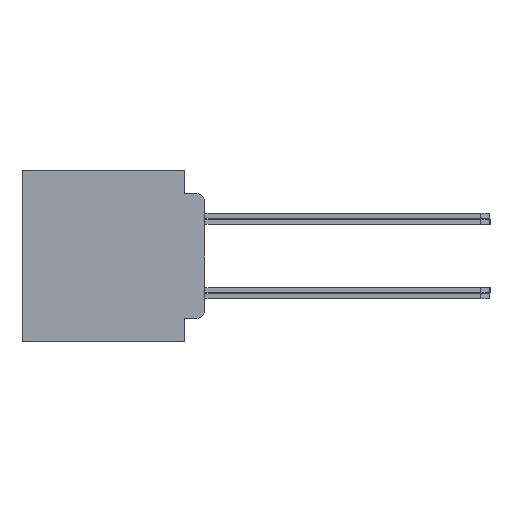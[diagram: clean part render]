
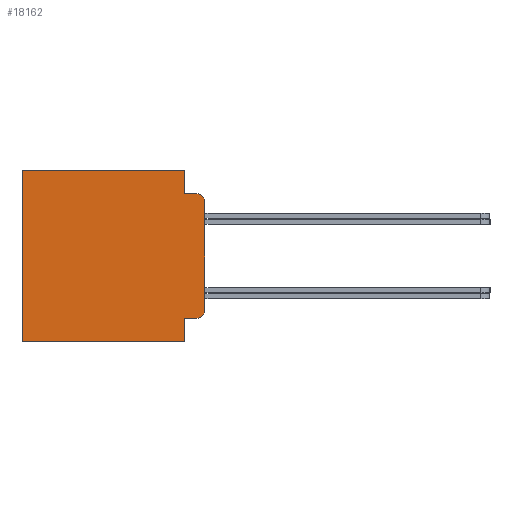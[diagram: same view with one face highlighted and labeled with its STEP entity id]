
A CAD part, left-side view. The second image highlights one B-rep face of the part: STEP entity #18162.
In plain terms, the highlighted planar face has unit normal (-1, 0, 0).
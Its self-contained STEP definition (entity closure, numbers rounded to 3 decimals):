
#563 = VERTEX_POINT ( 'NONE', #27452 ) ;
#600 = CARTESIAN_POINT ( 'NONE',  ( -67.462, 0., -5.486 ) ) ;
#1057 = EDGE_CURVE ( 'NONE', #22391, #24066, #13240, .T. ) ;
#1840 = LINE ( 'NONE', #24436, #25748 ) ;
#1884 = ORIENTED_EDGE ( 'NONE', *, *, #20820, .F. ) ;
#2280 = AXIS2_PLACEMENT_3D ( 'NONE', #17849, #24425, #22311 ) ;
#2644 = DIRECTION ( 'NONE',  ( 0., 1., 0. ) ) ;
#2706 = VERTEX_POINT ( 'NONE', #16538 ) ;
#3591 = LINE ( 'NONE', #10402, #8361 ) ;
#3735 = VECTOR ( 'NONE', #2644, 1000. ) ;
#3803 = AXIS2_PLACEMENT_3D ( 'NONE', #21195, #10219, #8195 ) ;
#3935 = CARTESIAN_POINT ( 'NONE',  ( -67.462, 1.295, 0. ) ) ;
#4358 = VERTEX_POINT ( 'NONE', #8052 ) ;
#4764 = ORIENTED_EDGE ( 'NONE', *, *, #26502, .T. ) ;
#4780 = ORIENTED_EDGE ( 'NONE', *, *, #1057, .F. ) ;
#5089 = CARTESIAN_POINT ( 'NONE',  ( -67.462, 0.508, -3.975 ) ) ;
#5610 = ORIENTED_EDGE ( 'NONE', *, *, #14342, .F. ) ;
#5852 = CIRCLE ( 'NONE', #2280, 0.508 ) ;
#6257 = ORIENTED_EDGE ( 'NONE', *, *, #21440, .F. ) ;
#6613 = CARTESIAN_POINT ( 'NONE',  ( -67.462, 11.684, -5.486 ) ) ;
#8052 = CARTESIAN_POINT ( 'NONE',  ( -67.462, 0., -3.467 ) ) ;
#8195 = DIRECTION ( 'NONE',  ( 0., 0., -1. ) ) ;
#8240 = VERTEX_POINT ( 'NONE', #24018 ) ;
#8361 = VECTOR ( 'NONE', #17074, 1000. ) ;
#8452 = VERTEX_POINT ( 'NONE', #5089 ) ;
#8797 = DIRECTION ( 'NONE',  ( 0., 0., -1. ) ) ;
#8942 = CARTESIAN_POINT ( 'NONE',  ( -67.462, 0., 5.486 ) ) ;
#9893 = CARTESIAN_POINT ( 'NONE',  ( -67.462, 1.295, -3.975 ) ) ;
#10219 = DIRECTION ( 'NONE',  ( 1., 0., 0. ) ) ;
#10402 = CARTESIAN_POINT ( 'NONE',  ( -67.462, 0., -5.486 ) ) ;
#10650 = CARTESIAN_POINT ( 'NONE',  ( -67.462, 1.295, 3.975 ) ) ;
#11885 = CARTESIAN_POINT ( 'NONE',  ( -67.462, 0.508, 3.975 ) ) ;
#11969 = FACE_OUTER_BOUND ( 'NONE', #21963, .T. ) ;
#12140 = VECTOR ( 'NONE', #8797, 1000. ) ;
#12455 = VERTEX_POINT ( 'NONE', #9893 ) ;
#13240 = LINE ( 'NONE', #600, #15978 ) ;
#13809 = LINE ( 'NONE', #3935, #17255 ) ;
#14342 = EDGE_CURVE ( 'NONE', #8240, #17278, #26118, .T. ) ;
#14702 = PLANE ( 'NONE',  #3803 ) ;
#14811 = DIRECTION ( 'NONE',  ( 0., 0., -1. ) ) ;
#14999 = EDGE_CURVE ( 'NONE', #2706, #17278, #18560, .T. ) ;
#15689 = ORIENTED_EDGE ( 'NONE', *, *, #21476, .T. ) ;
#15744 = ORIENTED_EDGE ( 'NONE', *, *, #24940, .F. ) ;
#15864 = DIRECTION ( 'NONE',  ( 0., 1., 0. ) ) ;
#15978 = VECTOR ( 'NONE', #15864, 1000. ) ;
#16538 = CARTESIAN_POINT ( 'NONE',  ( -67.462, 0., 3.467 ) ) ;
#16777 = ORIENTED_EDGE ( 'NONE', *, *, #14999, .T. ) ;
#17074 = DIRECTION ( 'NONE',  ( 0., 0., -1. ) ) ;
#17255 = VECTOR ( 'NONE', #17384, 1000. ) ;
#17278 = VERTEX_POINT ( 'NONE', #11885 ) ;
#17384 = DIRECTION ( 'NONE',  ( 0., 0., -1. ) ) ;
#17849 = CARTESIAN_POINT ( 'NONE',  ( -67.462, 0.508, -3.467 ) ) ;
#17924 = LINE ( 'NONE', #6613, #12140 ) ;
#18162 = ADVANCED_FACE ( 'NONE', ( #11969 ), #14702, .F. ) ;
#18242 = VECTOR ( 'NONE', #21243, 1000. ) ;
#18464 = EDGE_CURVE ( 'NONE', #563, #26416, #20806, .T. ) ;
#18560 = CIRCLE ( 'NONE', #24044, 0.508 ) ;
#18952 = VECTOR ( 'NONE', #26059, 1000. ) ;
#19640 = ORIENTED_EDGE ( 'NONE', *, *, #18464, .T. ) ;
#20806 = LINE ( 'NONE', #8942, #3735 ) ;
#20820 = EDGE_CURVE ( 'NONE', #563, #8240, #13809, .T. ) ;
#20874 = CARTESIAN_POINT ( 'NONE',  ( -67.462, 11.684, -5.486 ) ) ;
#21195 = CARTESIAN_POINT ( 'NONE',  ( -67.462, 0., -5.486 ) ) ;
#21243 = DIRECTION ( 'NONE',  ( 0., -1., 0. ) ) ;
#21440 = EDGE_CURVE ( 'NONE', #2706, #4358, #3591, .T. ) ;
#21476 = EDGE_CURVE ( 'NONE', #12455, #8452, #25810, .T. ) ;
#21943 = CARTESIAN_POINT ( 'NONE',  ( -67.462, 11.684, 5.486 ) ) ;
#21963 = EDGE_LOOP ( 'NONE', ( #15689, #4764, #6257, #16777, #5610, #1884, #19640, #23050, #4780, #15744 ) ) ;
#22311 = DIRECTION ( 'NONE',  ( 0., 0., -1. ) ) ;
#22391 = VERTEX_POINT ( 'NONE', #22645 ) ;
#22645 = CARTESIAN_POINT ( 'NONE',  ( -67.462, 1.295, -5.486 ) ) ;
#23050 = ORIENTED_EDGE ( 'NONE', *, *, #24404, .T. ) ;
#23775 = DIRECTION ( 'NONE',  ( -1., 0., 0. ) ) ;
#24018 = CARTESIAN_POINT ( 'NONE',  ( -67.462, 1.295, 3.975 ) ) ;
#24044 = AXIS2_PLACEMENT_3D ( 'NONE', #25886, #23775, #14811 ) ;
#24066 = VERTEX_POINT ( 'NONE', #20874 ) ;
#24404 = EDGE_CURVE ( 'NONE', #26416, #24066, #17924, .T. ) ;
#24425 = DIRECTION ( 'NONE',  ( -1., 0., 0. ) ) ;
#24436 = CARTESIAN_POINT ( 'NONE',  ( -67.462, 1.295, 0. ) ) ;
#24940 = EDGE_CURVE ( 'NONE', #12455, #22391, #1840, .T. ) ;
#25748 = VECTOR ( 'NONE', #26277, 1000. ) ;
#25810 = LINE ( 'NONE', #25957, #18952 ) ;
#25886 = CARTESIAN_POINT ( 'NONE',  ( -67.462, 0.508, 3.467 ) ) ;
#25957 = CARTESIAN_POINT ( 'NONE',  ( -67.462, 1.295, -3.975 ) ) ;
#26059 = DIRECTION ( 'NONE',  ( 0., -1., 0. ) ) ;
#26118 = LINE ( 'NONE', #10650, #18242 ) ;
#26277 = DIRECTION ( 'NONE',  ( 0., 0., -1. ) ) ;
#26416 = VERTEX_POINT ( 'NONE', #21943 ) ;
#26502 = EDGE_CURVE ( 'NONE', #8452, #4358, #5852, .T. ) ;
#27452 = CARTESIAN_POINT ( 'NONE',  ( -67.462, 1.295, 5.486 ) ) ;
